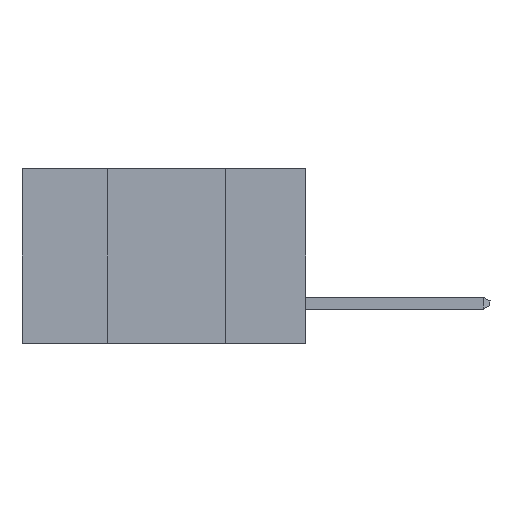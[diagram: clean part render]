
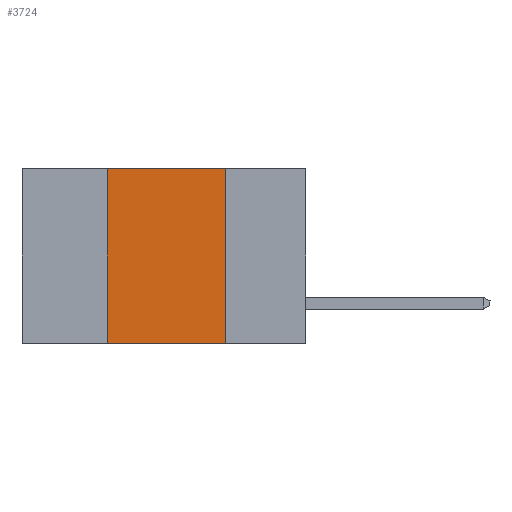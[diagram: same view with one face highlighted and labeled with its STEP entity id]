
A CAD part, left-side view. The second image highlights one B-rep face of the part: STEP entity #3724.
In plain terms, the highlighted planar face has unit normal (-1, 0, 0).
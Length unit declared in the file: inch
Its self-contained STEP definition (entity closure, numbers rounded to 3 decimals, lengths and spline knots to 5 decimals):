
#14 = AXIS2_PLACEMENT_3D ( 'NONE', #12244, #14342, #7082 ) ;
#425 = ORIENTED_EDGE ( 'NONE', *, *, #3840, .T. ) ;
#844 = LINE ( 'NONE', #7866, #6586 ) ;
#1035 = DIRECTION ( 'NONE',  ( 0., -1., 0. ) ) ;
#1793 = FACE_OUTER_BOUND ( 'NONE', #7044, .T. ) ;
#3121 = ORIENTED_EDGE ( 'NONE', *, *, #9418, .F. ) ;
#3724 = ADVANCED_FACE ( 'NONE', ( #1793 ), #8605, .F. ) ;
#3840 = EDGE_CURVE ( 'NONE', #6141, #15155, #14921, .T. ) ;
#4136 = DIRECTION ( 'NONE',  ( 0., 0., 1. ) ) ;
#4173 = VECTOR ( 'NONE', #21854, 39.37008 ) ;
#4548 = DIRECTION ( 'NONE',  ( 0., 0., -1. ) ) ;
#6141 = VERTEX_POINT ( 'NONE', #9480 ) ;
#6410 = VERTEX_POINT ( 'NONE', #19221 ) ;
#6586 = VECTOR ( 'NONE', #4136, 39.37008 ) ;
#6753 = CARTESIAN_POINT ( 'NONE',  ( 0., 0.17, -0.37 ) ) ;
#7044 = EDGE_LOOP ( 'NONE', ( #16666, #9233, #3121, #425 ) ) ;
#7082 = DIRECTION ( 'NONE',  ( 0., 0., -1. ) ) ;
#7581 = CARTESIAN_POINT ( 'NONE',  ( 0., 0.42, 0. ) ) ;
#7866 = CARTESIAN_POINT ( 'NONE',  ( 0., 0.42, -0.37 ) ) ;
#8395 = CARTESIAN_POINT ( 'NONE',  ( 0., 0.6, 0. ) ) ;
#8605 = PLANE ( 'NONE',  #14 ) ;
#9233 = ORIENTED_EDGE ( 'NONE', *, *, #14492, .F. ) ;
#9418 = EDGE_CURVE ( 'NONE', #6141, #19940, #844, .T. ) ;
#9480 = CARTESIAN_POINT ( 'NONE',  ( 0., 0.42, -0.37 ) ) ;
#10481 = EDGE_CURVE ( 'NONE', #6410, #15155, #22812, .T. ) ;
#11178 = CARTESIAN_POINT ( 'NONE',  ( 0., 0.6, -0.37 ) ) ;
#12244 = CARTESIAN_POINT ( 'NONE',  ( 0., 0.6, 0. ) ) ;
#13333 = VECTOR ( 'NONE', #4548, 39.37008 ) ;
#14342 = DIRECTION ( 'NONE',  ( 1., 0., 0. ) ) ;
#14492 = EDGE_CURVE ( 'NONE', #19940, #6410, #20379, .T. ) ;
#14921 = LINE ( 'NONE', #11178, #4173 ) ;
#15155 = VERTEX_POINT ( 'NONE', #16039 ) ;
#16039 = CARTESIAN_POINT ( 'NONE',  ( 0., 0.17, -0.37 ) ) ;
#16666 = ORIENTED_EDGE ( 'NONE', *, *, #10481, .F. ) ;
#17633 = VECTOR ( 'NONE', #1035, 39.37008 ) ;
#19221 = CARTESIAN_POINT ( 'NONE',  ( 0., 0.17, 0. ) ) ;
#19940 = VERTEX_POINT ( 'NONE', #7581 ) ;
#20379 = LINE ( 'NONE', #8395, #17633 ) ;
#21854 = DIRECTION ( 'NONE',  ( 0., -1., 0. ) ) ;
#22812 = LINE ( 'NONE', #6753, #13333 ) ;
